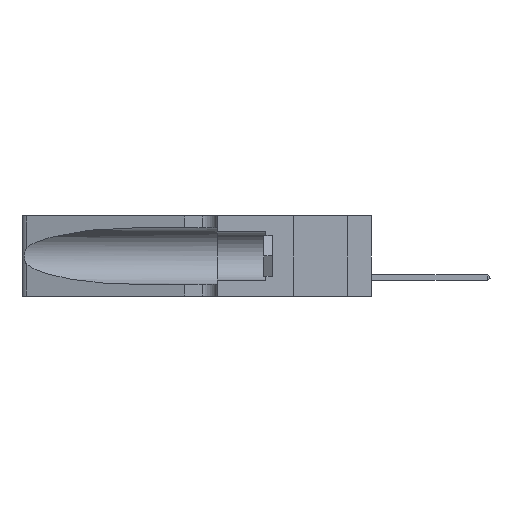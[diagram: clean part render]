
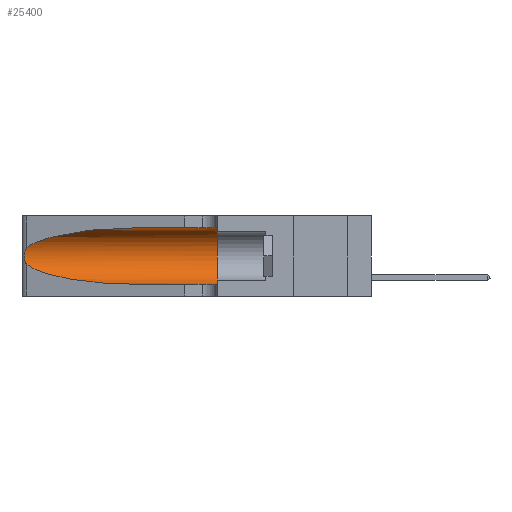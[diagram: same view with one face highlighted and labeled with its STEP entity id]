
A CAD part, left-side view. The second image highlights one B-rep face of the part: STEP entity #25400.
In plain terms, the highlighted cylindrical face has radius 3.308 mm (diameter 6.617 mm), a partial arc.
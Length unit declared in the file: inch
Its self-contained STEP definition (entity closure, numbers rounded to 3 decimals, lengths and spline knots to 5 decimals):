
#663 =( BOUNDED_CURVE ( )  B_SPLINE_CURVE ( 3, ( #25993, #38868, #9861, #1683 ),
 .UNSPECIFIED., .F., .F. ) 
 B_SPLINE_CURVE_WITH_KNOTS ( ( 4, 4 ),
 ( 3.44316, 4.71239 ),
 .UNSPECIFIED. ) 
 CURVE ( )  GEOMETRIC_REPRESENTATION_ITEM ( )  RATIONAL_B_SPLINE_CURVE ( ( 1., 0.87, 0.87, 1. ) ) 
 REPRESENTATION_ITEM ( '' )  );
#1556 = EDGE_CURVE ( 'NONE', #12833, #50059, #33971, .T. ) ;
#1683 = CARTESIAN_POINT ( 'NONE',  ( 0.1305, 0.72297, 0.05475 ) ) ;
#2101 = CARTESIAN_POINT ( 'NONE',  ( 0.25555, 1.22993, 0.14849 ) ) ;
#3821 = DIRECTION ( 'NONE',  ( 0., -1., 0. ) ) ;
#4425 = ORIENTED_EDGE ( 'NONE', *, *, #45722, .T. ) ;
#5420 = VECTOR ( 'NONE', #37037, 39.37008 ) ;
#6015 = CARTESIAN_POINT ( 'NONE',  ( 0.25639, 1.23184, 0.21858 ) ) ;
#7560 = DIRECTION ( 'NONE',  ( 0., 0., -1. ) ) ;
#7651 = CARTESIAN_POINT ( 'NONE',  ( 0.2373, 1.15595, 0.28018 ) ) ;
#9861 = CARTESIAN_POINT ( 'NONE',  ( 0.18966, 0.96281, 0.05475 ) ) ;
#9938 = CARTESIAN_POINT ( 'NONE',  ( 0.26017, 1.23833, 0.17102 ) ) ;
#12511 = AXIS2_PLACEMENT_3D ( 'NONE', #22921, #47369, #23084 ) ;
#12557 = CARTESIAN_POINT ( 'NONE',  ( 0.1305, 0.72297, 0.31525 ) ) ;
#12833 = VERTEX_POINT ( 'NONE', #16340 ) ;
#13141 = EDGE_CURVE ( 'NONE', #30275, #12833, #52222, .T. ) ;
#14030 = CARTESIAN_POINT ( 'NONE',  ( 0.25487, 1.22718, 0.14631 ) ) ;
#14199 = CARTESIAN_POINT ( 'NONE',  ( 0.25639, 1.23186, 0.15144 ) ) ;
#15031 = VERTEX_POINT ( 'NONE', #43015 ) ;
#15324 = CARTESIAN_POINT ( 'NONE',  ( 0.1305, 0.72297, 0.31525 ) ) ;
#15497 = EDGE_CURVE ( 'NONE', #44325, #15031, #663, .T. ) ;
#16057 = CARTESIAN_POINT ( 'NONE',  ( 0.1305, 0.35, 0.05475 ) ) ;
#16340 = CARTESIAN_POINT ( 'NONE',  ( 0.1305, 0.35, 0.31525 ) ) ;
#17419 = CARTESIAN_POINT ( 'NONE',  ( 0.1305, 1.61858, 0.05475 ) ) ;
#18584 = VERTEX_POINT ( 'NONE', #37474 ) ;
#19024 = EDGE_LOOP ( 'NONE', ( #22492, #4425, #33910, #21599, #42762, #51644 ) ) ;
#19900 = CARTESIAN_POINT ( 'NONE',  ( 0.25487, 1.22718, 0.22369 ) ) ;
#21599 = ORIENTED_EDGE ( 'NONE', *, *, #47489, .T. ) ;
#21769 = AXIS2_PLACEMENT_3D ( 'NONE', #24050, #3821, #7560 ) ;
#22044 = EDGE_CURVE ( 'NONE', #30275, #18584, #33492, .T. ) ;
#22315 = CARTESIAN_POINT ( 'NONE',  ( 0.26075, 1.23896, 0.19203 ) ) ;
#22492 = ORIENTED_EDGE ( 'NONE', *, *, #22044, .T. ) ;
#22921 = CARTESIAN_POINT ( 'NONE',  ( 0.1305, 0.35, 0.185 ) ) ;
#23084 = DIRECTION ( 'NONE',  ( 0., 0., 1. ) ) ;
#24050 = CARTESIAN_POINT ( 'NONE',  ( 0.1305, 1.61858, 0.185 ) ) ;
#25400 = ADVANCED_FACE ( 'NONE', ( #30477 ), #52008, .F. ) ;
#25993 = CARTESIAN_POINT ( 'NONE',  ( 0.25487, 1.22718, 0.14631 ) ) ;
#26234 = CARTESIAN_POINT ( 'NONE',  ( 0.25789, 1.23486, 0.15765 ) ) ;
#30161 = CARTESIAN_POINT ( 'NONE',  ( 0.26018, 1.23835, 0.19895 ) ) ;
#30275 = VERTEX_POINT ( 'NONE', #12557 ) ;
#30477 = FACE_OUTER_BOUND ( 'NONE', #19024, .T. ) ;
#33492 =( BOUNDED_CURVE ( )  B_SPLINE_CURVE ( 3, ( #15324, #48224, #7651, #19900 ),
 .UNSPECIFIED., .F., .T. ) 
 B_SPLINE_CURVE_WITH_KNOTS ( ( 4, 4 ),
 ( 1.5708, 2.84003 ),
 .UNSPECIFIED. ) 
 CURVE ( )  GEOMETRIC_REPRESENTATION_ITEM ( )  RATIONAL_B_SPLINE_CURVE ( ( 1., 0.87, 0.87, 1. ) ) 
 REPRESENTATION_ITEM ( '' )  );
#33876 = VECTOR ( 'NONE', #38860, 39.37008 ) ;
#33910 = ORIENTED_EDGE ( 'NONE', *, *, #15497, .T. ) ;
#33971 = CIRCLE ( 'NONE', #12511, 0.13025 ) ;
#34212 = CARTESIAN_POINT ( 'NONE',  ( 0.26075, 1.23896, 0.178 ) ) ;
#34371 = CARTESIAN_POINT ( 'NONE',  ( 0.25787, 1.23484, 0.2124 ) ) ;
#37037 = DIRECTION ( 'NONE',  ( 0., -1., 0. ) ) ;
#37474 = CARTESIAN_POINT ( 'NONE',  ( 0.25487, 1.22718, 0.22369 ) ) ;
#37760 = LINE ( 'NONE', #17419, #5420 ) ;
#38270 = CARTESIAN_POINT ( 'NONE',  ( 0.25856, 1.23593, 0.16098 ) ) ;
#38331 = B_SPLINE_CURVE_WITH_KNOTS ( 'NONE', 3,
 ( #42176, #38441, #6015, #34371, #50297, #30161, #22315, #34212, #9938, #38270, #26234, #14199, #2101, #14030 ),
 .UNSPECIFIED., .F., .F.,
 ( 4, 2, 2, 2, 2, 2, 4 ),
 ( 0., 0.00027, 0.00053, 0.00107, 0.0016, 0.00187, 0.00214 ),
 .UNSPECIFIED. ) ;
#38441 = CARTESIAN_POINT ( 'NONE',  ( 0.25555, 1.22994, 0.2215 ) ) ;
#38860 = DIRECTION ( 'NONE',  ( 0., -1., 0. ) ) ;
#38868 = CARTESIAN_POINT ( 'NONE',  ( 0.2373, 1.15595, 0.08982 ) ) ;
#42176 = CARTESIAN_POINT ( 'NONE',  ( 0.25487, 1.22718, 0.22369 ) ) ;
#42762 = ORIENTED_EDGE ( 'NONE', *, *, #1556, .F. ) ;
#43015 = CARTESIAN_POINT ( 'NONE',  ( 0.1305, 0.72297, 0.05475 ) ) ;
#44325 = VERTEX_POINT ( 'NONE', #49200 ) ;
#45722 = EDGE_CURVE ( 'NONE', #18584, #44325, #38331, .T. ) ;
#47026 = CARTESIAN_POINT ( 'NONE',  ( 0.1305, 1.61858, 0.31525 ) ) ;
#47369 = DIRECTION ( 'NONE',  ( 0., 1., 0. ) ) ;
#47489 = EDGE_CURVE ( 'NONE', #15031, #50059, #37760, .T. ) ;
#48224 = CARTESIAN_POINT ( 'NONE',  ( 0.18966, 0.96281, 0.31525 ) ) ;
#49200 = CARTESIAN_POINT ( 'NONE',  ( 0.25487, 1.22718, 0.14631 ) ) ;
#50059 = VERTEX_POINT ( 'NONE', #16057 ) ;
#50297 = CARTESIAN_POINT ( 'NONE',  ( 0.25854, 1.2359, 0.20912 ) ) ;
#51644 = ORIENTED_EDGE ( 'NONE', *, *, #13141, .F. ) ;
#52008 = CYLINDRICAL_SURFACE ( 'NONE', #21769, 0.13025 ) ;
#52222 = LINE ( 'NONE', #47026, #33876 ) ;
